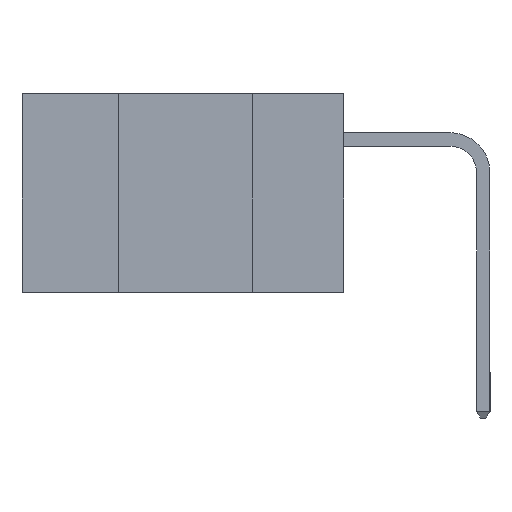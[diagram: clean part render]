
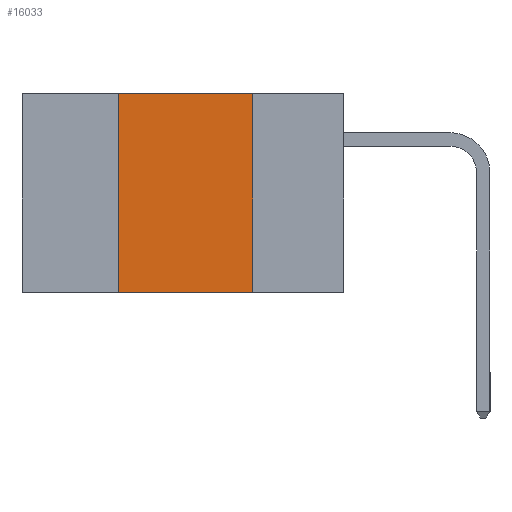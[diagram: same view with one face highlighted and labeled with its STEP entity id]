
A CAD part, left-side view. The second image highlights one B-rep face of the part: STEP entity #16033.
In plain terms, the highlighted planar face has unit normal (-1, 0, 0).
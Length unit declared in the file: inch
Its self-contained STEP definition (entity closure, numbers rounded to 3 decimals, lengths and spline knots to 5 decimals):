
#553 = VECTOR ( 'NONE', #18059, 39.37008 ) ;
#786 = VERTEX_POINT ( 'NONE', #15822 ) ;
#894 = DIRECTION ( 'NONE',  ( 0., -1., 0. ) ) ;
#898 = ORIENTED_EDGE ( 'NONE', *, *, #5509, .F. ) ;
#1020 = ORIENTED_EDGE ( 'NONE', *, *, #2808, .F. ) ;
#1367 = CARTESIAN_POINT ( 'NONE',  ( 0., 0.17, -0.37 ) ) ;
#1973 = AXIS2_PLACEMENT_3D ( 'NONE', #13454, #18300, #2549 ) ;
#2203 = VECTOR ( 'NONE', #14989, 39.37008 ) ;
#2447 = LINE ( 'NONE', #8683, #2203 ) ;
#2549 = DIRECTION ( 'NONE',  ( 0., 0., -1. ) ) ;
#2806 = LINE ( 'NONE', #5944, #5375 ) ;
#2808 = EDGE_CURVE ( 'NONE', #786, #12866, #16659, .T. ) ;
#2925 = CARTESIAN_POINT ( 'NONE',  ( 0., 0.42, -0.37 ) ) ;
#4459 = ORIENTED_EDGE ( 'NONE', *, *, #19369, .T. ) ;
#4703 = CARTESIAN_POINT ( 'NONE',  ( 0., 0.42, 0. ) ) ;
#5153 = VECTOR ( 'NONE', #894, 39.37008 ) ;
#5375 = VECTOR ( 'NONE', #9031, 39.37008 ) ;
#5509 = EDGE_CURVE ( 'NONE', #8801, #12498, #2806, .T. ) ;
#5944 = CARTESIAN_POINT ( 'NONE',  ( 0., 0.17, -0.37 ) ) ;
#7547 = PLANE ( 'NONE',  #1973 ) ;
#7636 = FACE_OUTER_BOUND ( 'NONE', #14697, .T. ) ;
#8683 = CARTESIAN_POINT ( 'NONE',  ( 0., 0.6, 0. ) ) ;
#8801 = VERTEX_POINT ( 'NONE', #13670 ) ;
#8867 = LINE ( 'NONE', #10194, #5153 ) ;
#9031 = DIRECTION ( 'NONE',  ( 0., 0., -1. ) ) ;
#10194 = CARTESIAN_POINT ( 'NONE',  ( 0., 0.6, -0.37 ) ) ;
#10297 = ORIENTED_EDGE ( 'NONE', *, *, #17688, .F. ) ;
#12498 = VERTEX_POINT ( 'NONE', #1367 ) ;
#12866 = VERTEX_POINT ( 'NONE', #4703 ) ;
#13454 = CARTESIAN_POINT ( 'NONE',  ( 0., 0.6, 0. ) ) ;
#13670 = CARTESIAN_POINT ( 'NONE',  ( 0., 0.17, 0. ) ) ;
#14697 = EDGE_LOOP ( 'NONE', ( #898, #10297, #1020, #4459 ) ) ;
#14989 = DIRECTION ( 'NONE',  ( 0., -1., 0. ) ) ;
#15822 = CARTESIAN_POINT ( 'NONE',  ( 0., 0.42, -0.37 ) ) ;
#16033 = ADVANCED_FACE ( 'NONE', ( #7636 ), #7547, .F. ) ;
#16659 = LINE ( 'NONE', #2925, #553 ) ;
#17688 = EDGE_CURVE ( 'NONE', #12866, #8801, #2447, .T. ) ;
#18059 = DIRECTION ( 'NONE',  ( 0., 0., 1. ) ) ;
#18300 = DIRECTION ( 'NONE',  ( 1., 0., 0. ) ) ;
#19369 = EDGE_CURVE ( 'NONE', #786, #12498, #8867, .T. ) ;
